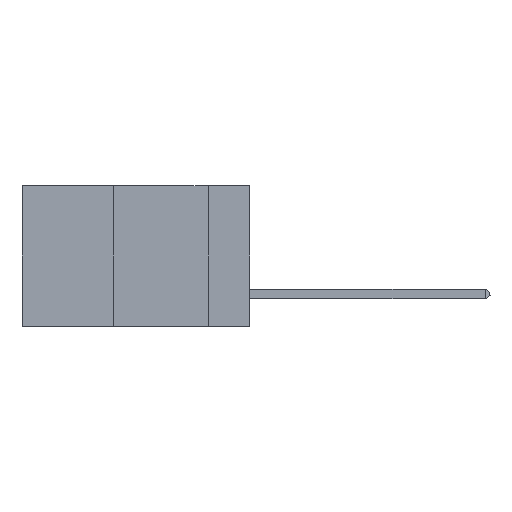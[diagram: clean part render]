
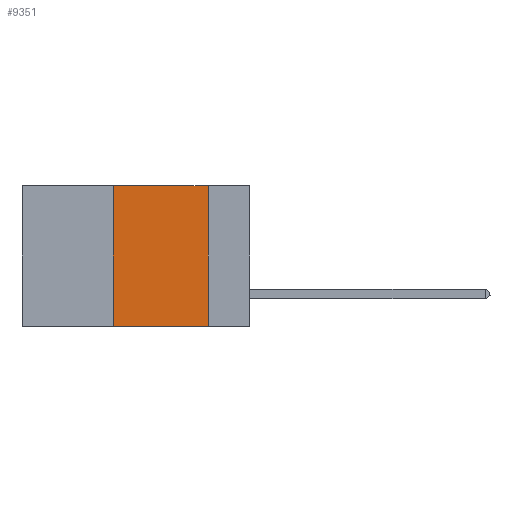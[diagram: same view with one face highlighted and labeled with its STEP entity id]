
A CAD part, left-side view. The second image highlights one B-rep face of the part: STEP entity #9351.
In plain terms, the highlighted planar face has unit normal (-1, 0, 0).
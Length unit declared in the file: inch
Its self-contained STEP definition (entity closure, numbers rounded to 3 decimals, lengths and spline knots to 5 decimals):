
#225 = DIRECTION ( 'NONE',  ( 1., 0., 0. ) ) ;
#467 = EDGE_CURVE ( 'NONE', #5409, #19844, #21008, .T. ) ;
#1971 = EDGE_CURVE ( 'NONE', #5409, #20624, #8267, .T. ) ;
#2673 = CARTESIAN_POINT ( 'NONE',  ( 0., 0.11, -0.37 ) ) ;
#2797 = VECTOR ( 'NONE', #18212, 39.37008 ) ;
#3869 = PLANE ( 'NONE',  #6162 ) ;
#5293 = ORIENTED_EDGE ( 'NONE', *, *, #11976, .F. ) ;
#5409 = VERTEX_POINT ( 'NONE', #7666 ) ;
#6036 = CARTESIAN_POINT ( 'NONE',  ( 0., 0.6, -0.37 ) ) ;
#6162 = AXIS2_PLACEMENT_3D ( 'NONE', #11967, #225, #17141 ) ;
#6831 = VERTEX_POINT ( 'NONE', #21609 ) ;
#7666 = CARTESIAN_POINT ( 'NONE',  ( 0., 0.36, -0.37 ) ) ;
#8267 = LINE ( 'NONE', #6036, #15899 ) ;
#8494 = ORIENTED_EDGE ( 'NONE', *, *, #1971, .T. ) ;
#9351 = ADVANCED_FACE ( 'NONE', ( #13680 ), #3869, .F. ) ;
#9662 = CARTESIAN_POINT ( 'NONE',  ( 0., 0.6, 0. ) ) ;
#9867 = DIRECTION ( 'NONE',  ( 0., -1., 0. ) ) ;
#10165 = CARTESIAN_POINT ( 'NONE',  ( 0., 0.36, 0. ) ) ;
#11340 = EDGE_LOOP ( 'NONE', ( #16575, #5293, #20140, #8494 ) ) ;
#11967 = CARTESIAN_POINT ( 'NONE',  ( 0., 0.6, 0. ) ) ;
#11976 = EDGE_CURVE ( 'NONE', #19844, #6831, #17683, .T. ) ;
#13269 = VECTOR ( 'NONE', #17259, 39.37008 ) ;
#13680 = FACE_OUTER_BOUND ( 'NONE', #11340, .T. ) ;
#14012 = CARTESIAN_POINT ( 'NONE',  ( 0., 0.11, 0. ) ) ;
#15899 = VECTOR ( 'NONE', #17829, 39.37008 ) ;
#16575 = ORIENTED_EDGE ( 'NONE', *, *, #19951, .F. ) ;
#16669 = CARTESIAN_POINT ( 'NONE',  ( 0., 0.36, 0. ) ) ;
#17141 = DIRECTION ( 'NONE',  ( 0., 0., -1. ) ) ;
#17259 = DIRECTION ( 'NONE',  ( 0., 0., -1. ) ) ;
#17683 = LINE ( 'NONE', #9662, #20551 ) ;
#17829 = DIRECTION ( 'NONE',  ( 0., -1., 0. ) ) ;
#18212 = DIRECTION ( 'NONE',  ( 0., 0., 1. ) ) ;
#18827 = LINE ( 'NONE', #14012, #13269 ) ;
#19844 = VERTEX_POINT ( 'NONE', #10165 ) ;
#19951 = EDGE_CURVE ( 'NONE', #6831, #20624, #18827, .T. ) ;
#20140 = ORIENTED_EDGE ( 'NONE', *, *, #467, .F. ) ;
#20551 = VECTOR ( 'NONE', #9867, 39.37008 ) ;
#20624 = VERTEX_POINT ( 'NONE', #2673 ) ;
#21008 = LINE ( 'NONE', #16669, #2797 ) ;
#21609 = CARTESIAN_POINT ( 'NONE',  ( 0., 0.11, 0. ) ) ;
